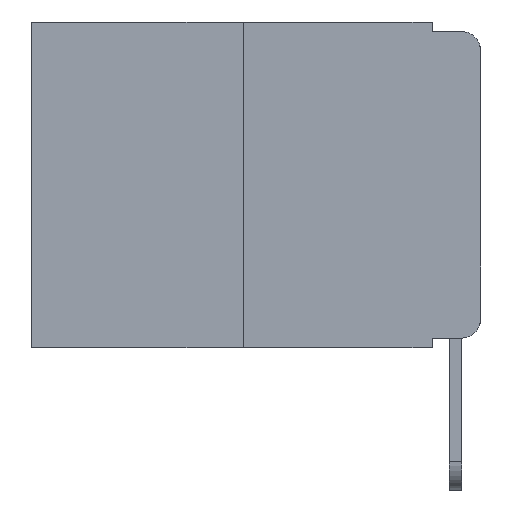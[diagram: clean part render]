
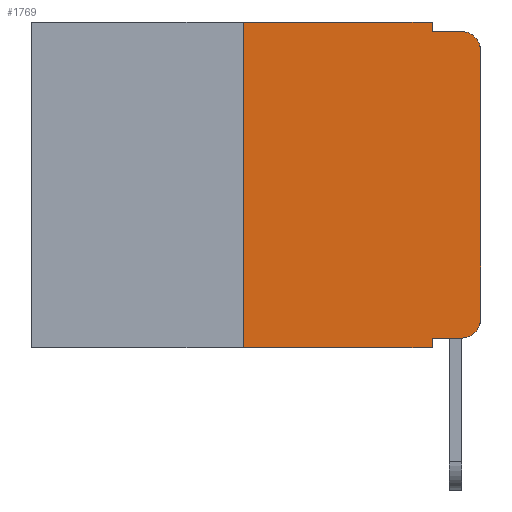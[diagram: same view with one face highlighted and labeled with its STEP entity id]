
A CAD part, left-side view. The second image highlights one B-rep face of the part: STEP entity #1769.
In plain terms, the highlighted planar face has unit normal (-1, 0, 0).
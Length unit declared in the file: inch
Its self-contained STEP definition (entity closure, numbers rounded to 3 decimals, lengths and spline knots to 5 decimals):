
#53 = EDGE_CURVE ( 'NONE', #3381, #8159, #487, .T. ) ;
#364 = LINE ( 'NONE', #9060, #2345 ) ;
#418 = CIRCLE ( 'NONE', #5684, 0.02 ) ;
#487 = LINE ( 'NONE', #6163, #7876 ) ;
#598 = VECTOR ( 'NONE', #2885, 39.37008 ) ;
#669 = CARTESIAN_POINT ( 'NONE',  ( 0., 0.051, -0.01 ) ) ;
#708 = LINE ( 'NONE', #9997, #6395 ) ;
#897 = CARTESIAN_POINT ( 'NONE',  ( 0., 0.25, 0. ) ) ;
#918 = ORIENTED_EDGE ( 'NONE', *, *, #10959, .T. ) ;
#1553 = ORIENTED_EDGE ( 'NONE', *, *, #6403, .T. ) ;
#1563 = VECTOR ( 'NONE', #9781, 39.37008 ) ;
#1769 = ADVANCED_FACE ( 'NONE', ( #11777 ), #8126, .F. ) ;
#1896 = VERTEX_POINT ( 'NONE', #897 ) ;
#1968 = VECTOR ( 'NONE', #7241, 39.37008 ) ;
#2070 = CARTESIAN_POINT ( 'NONE',  ( 0., 0.02, -0.333 ) ) ;
#2124 = LINE ( 'NONE', #11429, #1563 ) ;
#2345 = VECTOR ( 'NONE', #10024, 39.37008 ) ;
#2422 = VERTEX_POINT ( 'NONE', #3915 ) ;
#2704 = ORIENTED_EDGE ( 'NONE', *, *, #11025, .F. ) ;
#2708 = CARTESIAN_POINT ( 'NONE',  ( 0., 0.25, 0. ) ) ;
#2833 = ORIENTED_EDGE ( 'NONE', *, *, #6919, .T. ) ;
#2885 = DIRECTION ( 'NONE',  ( 0., 0., 1. ) ) ;
#3019 = DIRECTION ( 'NONE',  ( 0., 0., -1. ) ) ;
#3378 = CARTESIAN_POINT ( 'NONE',  ( 0., 0.051, -0.343 ) ) ;
#3381 = VERTEX_POINT ( 'NONE', #4794 ) ;
#3628 = EDGE_LOOP ( 'NONE', ( #8514, #918, #6101, #9464, #11619, #8932, #2833, #2704, #1553, #9381 ) ) ;
#3745 = CARTESIAN_POINT ( 'NONE',  ( 0., 0.051, -0.333 ) ) ;
#3769 = DIRECTION ( 'NONE',  ( -1., 0., 0. ) ) ;
#3904 = DIRECTION ( 'NONE',  ( 0., 0., 1. ) ) ;
#3915 = CARTESIAN_POINT ( 'NONE',  ( 0., 0.02, -0.01 ) ) ;
#4434 = EDGE_CURVE ( 'NONE', #1896, #3381, #708, .T. ) ;
#4513 = EDGE_CURVE ( 'NONE', #11293, #11184, #5689, .T. ) ;
#4748 = CARTESIAN_POINT ( 'NONE',  ( 0., 0., -0.03 ) ) ;
#4794 = CARTESIAN_POINT ( 'NONE',  ( 0., 0.051, 0. ) ) ;
#4909 = EDGE_CURVE ( 'NONE', #5347, #1896, #5700, .T. ) ;
#5133 = CARTESIAN_POINT ( 'NONE',  ( 0., 0.473, 0. ) ) ;
#5347 = VERTEX_POINT ( 'NONE', #7260 ) ;
#5646 = CARTESIAN_POINT ( 'NONE',  ( 0., 0.02, -0.03 ) ) ;
#5684 = AXIS2_PLACEMENT_3D ( 'NONE', #5646, #9327, #7393 ) ;
#5689 = CIRCLE ( 'NONE', #7429, 0.02 ) ;
#5700 = LINE ( 'NONE', #2708, #598 ) ;
#5785 = CARTESIAN_POINT ( 'NONE',  ( 0., 0., 0. ) ) ;
#5862 = VECTOR ( 'NONE', #3019, 39.37008 ) ;
#6101 = ORIENTED_EDGE ( 'NONE', *, *, #11465, .F. ) ;
#6163 = CARTESIAN_POINT ( 'NONE',  ( 0., 0.051, 0. ) ) ;
#6395 = VECTOR ( 'NONE', #7104, 39.37008 ) ;
#6403 = EDGE_CURVE ( 'NONE', #7898, #11293, #364, .T. ) ;
#6910 = LINE ( 'NONE', #10529, #5862 ) ;
#6919 = EDGE_CURVE ( 'NONE', #5347, #7782, #9046, .T. ) ;
#7104 = DIRECTION ( 'NONE',  ( 0., -1., 0. ) ) ;
#7241 = DIRECTION ( 'NONE',  ( 0., -1., 0. ) ) ;
#7260 = CARTESIAN_POINT ( 'NONE',  ( 0., 0.25, -0.343 ) ) ;
#7336 = CARTESIAN_POINT ( 'NONE',  ( 0., 0.02, -0.313 ) ) ;
#7393 = DIRECTION ( 'NONE',  ( 0., 0., -1. ) ) ;
#7429 = AXIS2_PLACEMENT_3D ( 'NONE', #7336, #3769, #11032 ) ;
#7782 = VERTEX_POINT ( 'NONE', #3378 ) ;
#7876 = VECTOR ( 'NONE', #9051, 39.37008 ) ;
#7898 = VERTEX_POINT ( 'NONE', #3745 ) ;
#8018 = DIRECTION ( 'NONE',  ( 0., 0., -1. ) ) ;
#8126 = PLANE ( 'NONE',  #10692 ) ;
#8130 = CARTESIAN_POINT ( 'NONE',  ( 0., 0.473, -0.343 ) ) ;
#8159 = VERTEX_POINT ( 'NONE', #669 ) ;
#8514 = ORIENTED_EDGE ( 'NONE', *, *, #11802, .T. ) ;
#8932 = ORIENTED_EDGE ( 'NONE', *, *, #4909, .F. ) ;
#9046 = LINE ( 'NONE', #8130, #1968 ) ;
#9051 = DIRECTION ( 'NONE',  ( 0., 0., -1. ) ) ;
#9060 = CARTESIAN_POINT ( 'NONE',  ( 0., 0.051, -0.333 ) ) ;
#9287 = LINE ( 'NONE', #5785, #10283 ) ;
#9327 = DIRECTION ( 'NONE',  ( -1., 0., 0. ) ) ;
#9381 = ORIENTED_EDGE ( 'NONE', *, *, #4513, .T. ) ;
#9464 = ORIENTED_EDGE ( 'NONE', *, *, #53, .F. ) ;
#9781 = DIRECTION ( 'NONE',  ( 0., -1., 0. ) ) ;
#9997 = CARTESIAN_POINT ( 'NONE',  ( 0., 0.473, 0. ) ) ;
#10024 = DIRECTION ( 'NONE',  ( 0., -1., 0. ) ) ;
#10029 = VERTEX_POINT ( 'NONE', #4748 ) ;
#10283 = VECTOR ( 'NONE', #3904, 39.37008 ) ;
#10529 = CARTESIAN_POINT ( 'NONE',  ( 0., 0.051, 0. ) ) ;
#10692 = AXIS2_PLACEMENT_3D ( 'NONE', #5133, #11594, #8018 ) ;
#10959 = EDGE_CURVE ( 'NONE', #10029, #2422, #418, .T. ) ;
#11025 = EDGE_CURVE ( 'NONE', #7898, #7782, #6910, .T. ) ;
#11032 = DIRECTION ( 'NONE',  ( 0., 0., -1. ) ) ;
#11184 = VERTEX_POINT ( 'NONE', #11753 ) ;
#11293 = VERTEX_POINT ( 'NONE', #2070 ) ;
#11429 = CARTESIAN_POINT ( 'NONE',  ( 0., 0.051, -0.01 ) ) ;
#11465 = EDGE_CURVE ( 'NONE', #8159, #2422, #2124, .T. ) ;
#11594 = DIRECTION ( 'NONE',  ( 1., 0., 0. ) ) ;
#11619 = ORIENTED_EDGE ( 'NONE', *, *, #4434, .F. ) ;
#11753 = CARTESIAN_POINT ( 'NONE',  ( 0., 0., -0.313 ) ) ;
#11777 = FACE_OUTER_BOUND ( 'NONE', #3628, .T. ) ;
#11802 = EDGE_CURVE ( 'NONE', #11184, #10029, #9287, .T. ) ;
